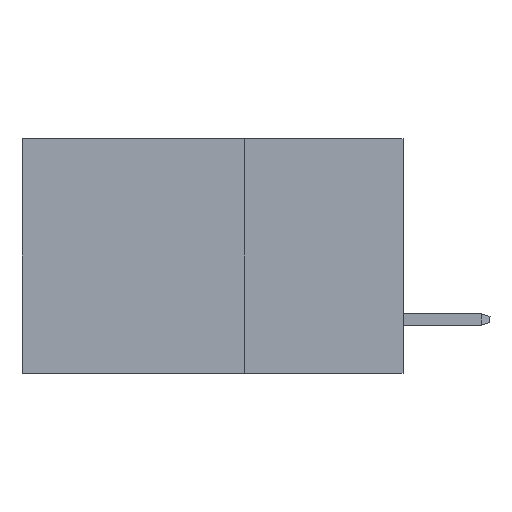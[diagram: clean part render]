
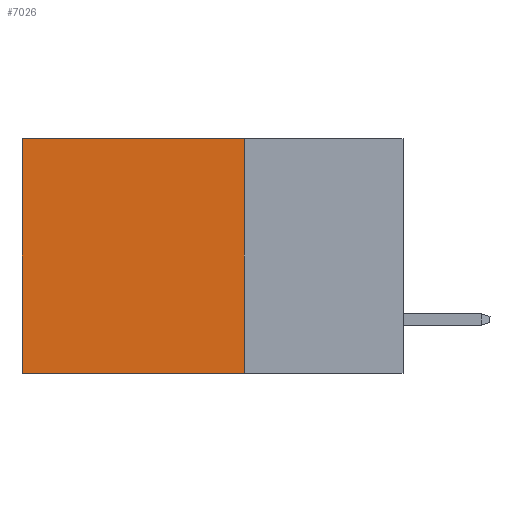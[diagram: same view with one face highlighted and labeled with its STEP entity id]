
A CAD part, left-side view. The second image highlights one B-rep face of the part: STEP entity #7026.
In plain terms, the highlighted planar face has unit normal (-1, 0, 0).
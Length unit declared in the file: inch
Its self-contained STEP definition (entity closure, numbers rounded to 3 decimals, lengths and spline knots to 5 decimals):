
#70 = EDGE_CURVE ( 'NONE', #5289, #7406, #6574, .T. ) ;
#271 = EDGE_LOOP ( 'NONE', ( #8861, #3278, #6113, #6406 ) ) ;
#841 = VERTEX_POINT ( 'NONE', #1491 ) ;
#1313 = CARTESIAN_POINT ( 'NONE',  ( 0.2875, 0.25, 0. ) ) ;
#1455 = LINE ( 'NONE', #5851, #1677 ) ;
#1491 = CARTESIAN_POINT ( 'NONE',  ( 0.2875, 0.6, -0.37 ) ) ;
#1624 = VECTOR ( 'NONE', #8561, 39.37008 ) ;
#1677 = VECTOR ( 'NONE', #5894, 39.37008 ) ;
#1763 = VECTOR ( 'NONE', #5161, 39.37008 ) ;
#2002 = AXIS2_PLACEMENT_3D ( 'NONE', #5007, #9610, #6570 ) ;
#2087 = LINE ( 'NONE', #4495, #1763 ) ;
#2486 = LINE ( 'NONE', #3239, #1624 ) ;
#3239 = CARTESIAN_POINT ( 'NONE',  ( 0.2875, 0.6, 0. ) ) ;
#3278 = ORIENTED_EDGE ( 'NONE', *, *, #7613, .F. ) ;
#3630 = DIRECTION ( 'NONE',  ( 0., 1., 0. ) ) ;
#3821 = VECTOR ( 'NONE', #3630, 39.37008 ) ;
#4495 = CARTESIAN_POINT ( 'NONE',  ( 0.2875, 0.25, 0. ) ) ;
#5007 = CARTESIAN_POINT ( 'NONE',  ( 0.2875, 0.25, 0. ) ) ;
#5161 = DIRECTION ( 'NONE',  ( 0., 0., -1. ) ) ;
#5289 = VERTEX_POINT ( 'NONE', #7703 ) ;
#5424 = EDGE_CURVE ( 'NONE', #7406, #841, #2486, .T. ) ;
#5851 = CARTESIAN_POINT ( 'NONE',  ( 0.2875, 0.25, -0.37 ) ) ;
#5861 = FACE_OUTER_BOUND ( 'NONE', #271, .T. ) ;
#5894 = DIRECTION ( 'NONE',  ( 0., 1., 0. ) ) ;
#5914 = CARTESIAN_POINT ( 'NONE',  ( 0.2875, 0.25, -0.37 ) ) ;
#6113 = ORIENTED_EDGE ( 'NONE', *, *, #9543, .F. ) ;
#6406 = ORIENTED_EDGE ( 'NONE', *, *, #70, .T. ) ;
#6570 = DIRECTION ( 'NONE',  ( 0., 0., -1. ) ) ;
#6574 = LINE ( 'NONE', #1313, #3821 ) ;
#7018 = CARTESIAN_POINT ( 'NONE',  ( 0.2875, 0.6, 0. ) ) ;
#7026 = ADVANCED_FACE ( 'NONE', ( #5861 ), #8088, .F. ) ;
#7406 = VERTEX_POINT ( 'NONE', #7018 ) ;
#7613 = EDGE_CURVE ( 'NONE', #7915, #841, #1455, .T. ) ;
#7703 = CARTESIAN_POINT ( 'NONE',  ( 0.2875, 0.25, 0. ) ) ;
#7915 = VERTEX_POINT ( 'NONE', #5914 ) ;
#8088 = PLANE ( 'NONE',  #2002 ) ;
#8561 = DIRECTION ( 'NONE',  ( 0., 0., -1. ) ) ;
#8861 = ORIENTED_EDGE ( 'NONE', *, *, #5424, .T. ) ;
#9543 = EDGE_CURVE ( 'NONE', #5289, #7915, #2087, .T. ) ;
#9610 = DIRECTION ( 'NONE',  ( 1., 0., 0. ) ) ;
